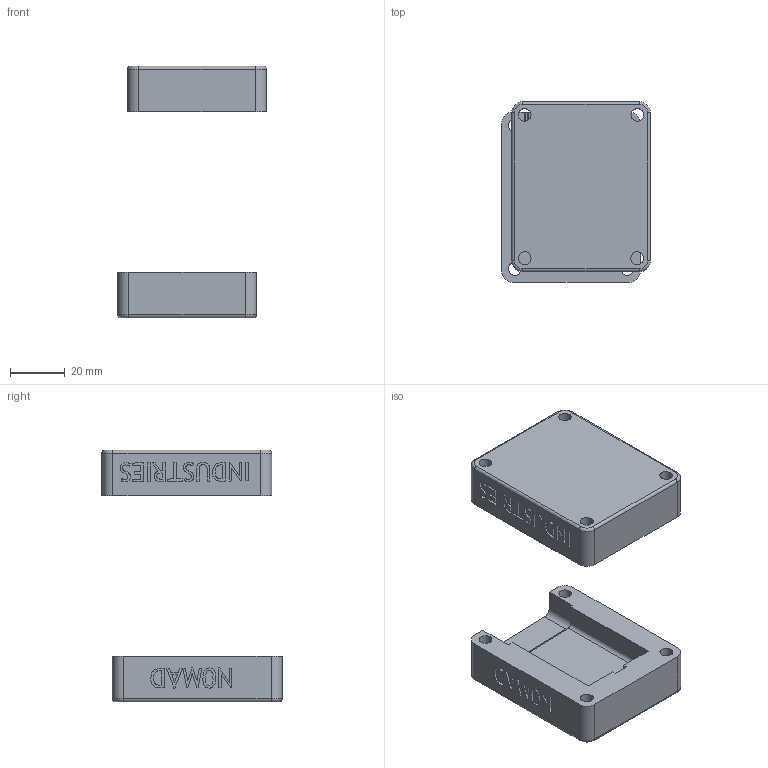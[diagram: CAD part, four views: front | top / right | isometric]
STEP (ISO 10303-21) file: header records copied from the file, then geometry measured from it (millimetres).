
FILE_DESCRIPTION(/* description */ (''),/* implementation_level */ '2;1');
FILE_NAME(/* name */ 'Madsen magazine extension Short v8.step',/* time_stamp */ '2018-09-18T20:20:33-05:00',/* author */ ('greg.bestland'),/* organization */ (''),/* preprocessor_version */ 'ST-DEVELOPER v17.2',/* originating_system */ 'Autodesk Translation Framework v7.6.0.251',/* authorisation */ '');
FILE_SCHEMA (('AUTOMOTIVE_DESIGN { 1 0 10303 214 3 1 1 }'));
Length unit declared in the file: millimetre
Products named in the file (1): Madsen magazine extension Short
Bounding box: 54.28 x 65.74 x 91.75 mm (x, y, z)
Volume: 68833 mm3; surface area: 24052.9 mm2
Topology: 2 solids, 2 shells, 468 faces, 1270 edges, 839 vertices
Faces by surface type: plane 267, bspline 155, cylinder 38, torus 8
Full cylindrical faces by diameter (mm): 4.6 x4
Entity records: 16088 total; most frequent: CARTESIAN_POINT 5213, ORIENTED_EDGE 2540, DIRECTION 1672, EDGE_CURVE 1270, LINE 876, VECTOR 876, VERTEX_POINT 839, EDGE_LOOP 517
